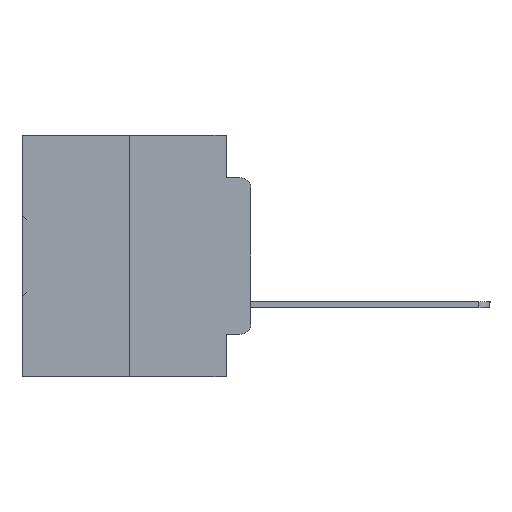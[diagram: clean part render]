
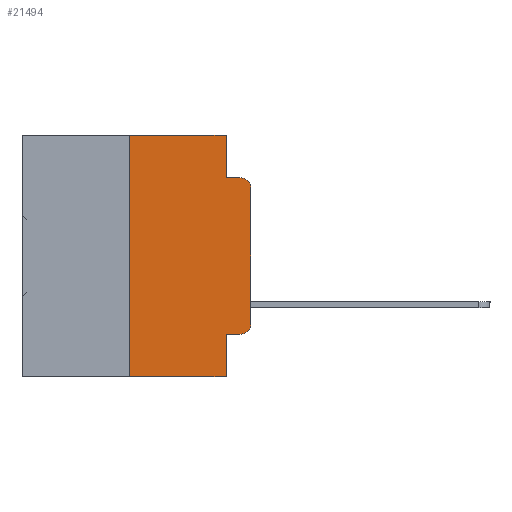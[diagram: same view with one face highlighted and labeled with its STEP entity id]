
A CAD part, left-side view. The second image highlights one B-rep face of the part: STEP entity #21494.
In plain terms, the highlighted planar face has unit normal (-1, 0, 0).
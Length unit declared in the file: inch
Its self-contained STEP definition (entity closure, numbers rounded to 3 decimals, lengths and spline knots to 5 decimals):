
#78 = VECTOR ( 'NONE', #10063, 39.37008 ) ;
#248 = EDGE_CURVE ( 'NONE', #34295, #6870, #21934, .T. ) ;
#750 = VECTOR ( 'NONE', #25041, 39.37008 ) ;
#946 = LINE ( 'NONE', #17171, #9027 ) ;
#1550 = VERTEX_POINT ( 'NONE', #8620 ) ;
#1627 = VERTEX_POINT ( 'NONE', #11696 ) ;
#1688 = CARTESIAN_POINT ( 'NONE',  ( 0., 0.25, 0. ) ) ;
#2404 = CARTESIAN_POINT ( 'NONE',  ( 0., 0.051, -0.0885 ) ) ;
#2629 = CIRCLE ( 'NONE', #9676, 0.02 ) ;
#2718 = PLANE ( 'NONE',  #10055 ) ;
#3073 = EDGE_CURVE ( 'NONE', #6870, #1627, #2629, .T. ) ;
#4018 = VECTOR ( 'NONE', #19982, 39.37008 ) ;
#5005 = CARTESIAN_POINT ( 'NONE',  ( 0., 0.02, -0.3915 ) ) ;
#5562 = ORIENTED_EDGE ( 'NONE', *, *, #30012, .T. ) ;
#5927 = LINE ( 'NONE', #28146, #4018 ) ;
#6612 = ORIENTED_EDGE ( 'NONE', *, *, #26834, .F. ) ;
#6847 = EDGE_CURVE ( 'NONE', #34083, #30090, #5927, .T. ) ;
#6870 = VERTEX_POINT ( 'NONE', #10440 ) ;
#7964 = EDGE_CURVE ( 'NONE', #1550, #30403, #946, .T. ) ;
#8027 = VECTOR ( 'NONE', #9789, 39.37008 ) ;
#8076 = CARTESIAN_POINT ( 'NONE',  ( 0., 0.051, -0.4115 ) ) ;
#8294 = VECTOR ( 'NONE', #27570, 39.37008 ) ;
#8546 = DIRECTION ( 'NONE',  ( 1., 0., 0. ) ) ;
#8620 = CARTESIAN_POINT ( 'NONE',  ( 0., 0.25, -0.5 ) ) ;
#9027 = VECTOR ( 'NONE', #14602, 39.37008 ) ;
#9455 = CARTESIAN_POINT ( 'NONE',  ( 0., 0.051, -0.4115 ) ) ;
#9676 = AXIS2_PLACEMENT_3D ( 'NONE', #5005, #27583, #16149 ) ;
#9789 = DIRECTION ( 'NONE',  ( 0., -1., 0. ) ) ;
#10055 = AXIS2_PLACEMENT_3D ( 'NONE', #25292, #8546, #19493 ) ;
#10063 = DIRECTION ( 'NONE',  ( 0., -1., 0. ) ) ;
#10440 = CARTESIAN_POINT ( 'NONE',  ( 0., 0.02, -0.4115 ) ) ;
#10511 = EDGE_CURVE ( 'NONE', #1550, #16528, #32288, .T. ) ;
#11061 = CARTESIAN_POINT ( 'NONE',  ( 0., 0.02, -0.1085 ) ) ;
#11696 = CARTESIAN_POINT ( 'NONE',  ( 0., 0., -0.3915 ) ) ;
#12691 = EDGE_LOOP ( 'NONE', ( #5562, #31670, #13957, #24263, #6612, #13250, #15237, #25851, #13617, #14870 ) ) ;
#12972 = CARTESIAN_POINT ( 'NONE',  ( 0., 0.02, -0.0885 ) ) ;
#13250 = ORIENTED_EDGE ( 'NONE', *, *, #7964, .F. ) ;
#13316 = CARTESIAN_POINT ( 'NONE',  ( 0., 0.051, 0. ) ) ;
#13413 = CARTESIAN_POINT ( 'NONE',  ( 0., 0.051, 0. ) ) ;
#13526 = LINE ( 'NONE', #2404, #17277 ) ;
#13617 = ORIENTED_EDGE ( 'NONE', *, *, #248, .T. ) ;
#13957 = ORIENTED_EDGE ( 'NONE', *, *, #25678, .F. ) ;
#14602 = DIRECTION ( 'NONE',  ( 0., 0., 1. ) ) ;
#14870 = ORIENTED_EDGE ( 'NONE', *, *, #3073, .T. ) ;
#15237 = ORIENTED_EDGE ( 'NONE', *, *, #10511, .T. ) ;
#15774 = CARTESIAN_POINT ( 'NONE',  ( 0., 0., 0. ) ) ;
#16036 = DIRECTION ( 'NONE',  ( -1., 0., 0. ) ) ;
#16149 = DIRECTION ( 'NONE',  ( 0., 0., -1. ) ) ;
#16528 = VERTEX_POINT ( 'NONE', #26512 ) ;
#17001 = CARTESIAN_POINT ( 'NONE',  ( 0., 0., -0.1085 ) ) ;
#17171 = CARTESIAN_POINT ( 'NONE',  ( 0., 0.25, 0. ) ) ;
#17277 = VECTOR ( 'NONE', #24625, 39.37008 ) ;
#19493 = DIRECTION ( 'NONE',  ( 0., 0., -1. ) ) ;
#19982 = DIRECTION ( 'NONE',  ( 0., 0., -1. ) ) ;
#20719 = LINE ( 'NONE', #34744, #8027 ) ;
#20995 = CARTESIAN_POINT ( 'NONE',  ( 0., 0.473, -0.5 ) ) ;
#21494 = ADVANCED_FACE ( 'NONE', ( #30412 ), #2718, .F. ) ;
#21934 = LINE ( 'NONE', #8076, #8294 ) ;
#22715 = VECTOR ( 'NONE', #24296, 39.37008 ) ;
#24263 = ORIENTED_EDGE ( 'NONE', *, *, #6847, .F. ) ;
#24296 = DIRECTION ( 'NONE',  ( 0., 0., 1. ) ) ;
#24625 = DIRECTION ( 'NONE',  ( 0., -1., 0. ) ) ;
#24996 = CARTESIAN_POINT ( 'NONE',  ( 0., 0.051, -0.0885 ) ) ;
#25041 = DIRECTION ( 'NONE',  ( 0., 0., -1. ) ) ;
#25292 = CARTESIAN_POINT ( 'NONE',  ( 0., 0.473, 0. ) ) ;
#25678 = EDGE_CURVE ( 'NONE', #30090, #30415, #13526, .T. ) ;
#25851 = ORIENTED_EDGE ( 'NONE', *, *, #30790, .F. ) ;
#26512 = CARTESIAN_POINT ( 'NONE',  ( 0., 0.051, -0.5 ) ) ;
#26834 = EDGE_CURVE ( 'NONE', #30403, #34083, #20719, .T. ) ;
#27130 = DIRECTION ( 'NONE',  ( 0., 0., -1. ) ) ;
#27570 = DIRECTION ( 'NONE',  ( 0., -1., 0. ) ) ;
#27583 = DIRECTION ( 'NONE',  ( -1., 0., 0. ) ) ;
#27789 = LINE ( 'NONE', #13413, #750 ) ;
#27937 = EDGE_CURVE ( 'NONE', #31459, #30415, #33080, .T. ) ;
#28146 = CARTESIAN_POINT ( 'NONE',  ( 0., 0.051, 0. ) ) ;
#30012 = EDGE_CURVE ( 'NONE', #1627, #31459, #30133, .T. ) ;
#30090 = VERTEX_POINT ( 'NONE', #24996 ) ;
#30133 = LINE ( 'NONE', #15774, #22715 ) ;
#30403 = VERTEX_POINT ( 'NONE', #1688 ) ;
#30412 = FACE_OUTER_BOUND ( 'NONE', #12691, .T. ) ;
#30415 = VERTEX_POINT ( 'NONE', #12972 ) ;
#30790 = EDGE_CURVE ( 'NONE', #34295, #16528, #27789, .T. ) ;
#31459 = VERTEX_POINT ( 'NONE', #17001 ) ;
#31670 = ORIENTED_EDGE ( 'NONE', *, *, #27937, .T. ) ;
#31928 = AXIS2_PLACEMENT_3D ( 'NONE', #11061, #16036, #27130 ) ;
#32288 = LINE ( 'NONE', #20995, #78 ) ;
#33080 = CIRCLE ( 'NONE', #31928, 0.02 ) ;
#34083 = VERTEX_POINT ( 'NONE', #13316 ) ;
#34295 = VERTEX_POINT ( 'NONE', #9455 ) ;
#34744 = CARTESIAN_POINT ( 'NONE',  ( 0., 0.473, 0. ) ) ;
